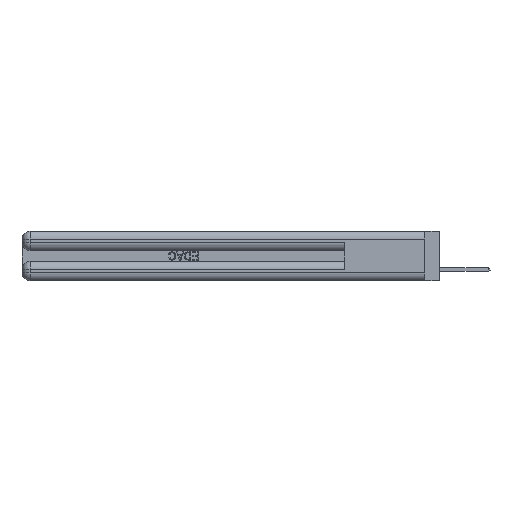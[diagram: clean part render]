
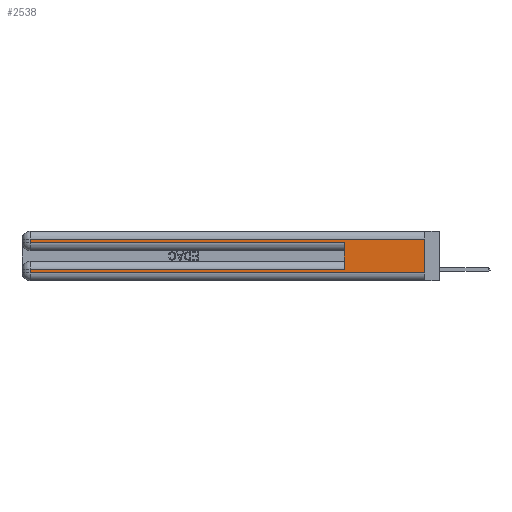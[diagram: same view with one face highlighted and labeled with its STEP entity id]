
A CAD part, left-side view. The second image highlights one B-rep face of the part: STEP entity #2538.
In plain terms, the highlighted planar face has unit normal (-1, 0, 0).
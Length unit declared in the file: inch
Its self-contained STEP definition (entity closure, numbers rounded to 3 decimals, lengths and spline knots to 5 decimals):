
#1200 = CARTESIAN_POINT ( 'NONE',  ( 0., 0., 0.37 ) ) ;
#1521 = CARTESIAN_POINT ( 'NONE',  ( 0., 0.6, 0.285 ) ) ;
#2370 = AXIS2_PLACEMENT_3D ( 'NONE', #34745, #12006, #21709 ) ;
#2538 = ADVANCED_FACE ( 'NONE', ( #9168 ), #5269, .F. ) ;
#3090 = DIRECTION ( 'NONE',  ( 0., 0., -1. ) ) ;
#3160 = DIRECTION ( 'NONE',  ( 0., 1., 0. ) ) ;
#3870 = DIRECTION ( 'NONE',  ( 0., -1., 0. ) ) ;
#5269 = PLANE ( 'NONE',  #2370 ) ;
#5650 = EDGE_CURVE ( 'NONE', #10158, #11535, #15605, .T. ) ;
#6093 = VECTOR ( 'NONE', #3160, 39.37008 ) ;
#6215 = LINE ( 'NONE', #7776, #11859 ) ;
#6504 = LINE ( 'NONE', #20727, #42421 ) ;
#6825 = VERTEX_POINT ( 'NONE', #21568 ) ;
#7388 = DIRECTION ( 'NONE',  ( 0., 1., 0. ) ) ;
#7776 = CARTESIAN_POINT ( 'NONE',  ( 0., 0.6, 0.145 ) ) ;
#9168 = FACE_OUTER_BOUND ( 'NONE', #27084, .T. ) ;
#10158 = VERTEX_POINT ( 'NONE', #32907 ) ;
#10251 = EDGE_CURVE ( 'NONE', #6825, #13430, #14712, .T. ) ;
#10540 = CARTESIAN_POINT ( 'NONE',  ( 0., 2.94, 0.37 ) ) ;
#10787 = CARTESIAN_POINT ( 'NONE',  ( 0., 2.94, 0.31 ) ) ;
#11535 = VERTEX_POINT ( 'NONE', #21443 ) ;
#11615 = DIRECTION ( 'NONE',  ( 0., -1., 0. ) ) ;
#11859 = VECTOR ( 'NONE', #14200, 39.37008 ) ;
#11925 = EDGE_CURVE ( 'NONE', #23346, #28548, #39711, .T. ) ;
#12006 = DIRECTION ( 'NONE',  ( 1., 0., 0. ) ) ;
#12674 = VERTEX_POINT ( 'NONE', #24834 ) ;
#13420 = EDGE_CURVE ( 'NONE', #23346, #11535, #28756, .T. ) ;
#13430 = VERTEX_POINT ( 'NONE', #1521 ) ;
#13829 = EDGE_CURVE ( 'NONE', #41692, #13430, #6215, .T. ) ;
#14200 = DIRECTION ( 'NONE',  ( 0., 0., 1. ) ) ;
#14659 = ORIENTED_EDGE ( 'NONE', *, *, #29208, .T. ) ;
#14712 = LINE ( 'NONE', #39731, #20286 ) ;
#15605 = LINE ( 'NONE', #37679, #32944 ) ;
#15914 = ORIENTED_EDGE ( 'NONE', *, *, #23931, .T. ) ;
#20286 = VECTOR ( 'NONE', #3870, 39.37008 ) ;
#20727 = CARTESIAN_POINT ( 'NONE',  ( 0., 2.94, 0.37 ) ) ;
#21443 = CARTESIAN_POINT ( 'NONE',  ( 0., 0., 0.06 ) ) ;
#21556 = VECTOR ( 'NONE', #3090, 39.37008 ) ;
#21568 = CARTESIAN_POINT ( 'NONE',  ( 0., 2.94, 0.285 ) ) ;
#21709 = DIRECTION ( 'NONE',  ( 0., 0., -1. ) ) ;
#22285 = VECTOR ( 'NONE', #7388, 39.37008 ) ;
#23346 = VERTEX_POINT ( 'NONE', #38727 ) ;
#23931 = EDGE_CURVE ( 'NONE', #28548, #6825, #6504, .T. ) ;
#24834 = CARTESIAN_POINT ( 'NONE',  ( 0., 2.94, 0.085 ) ) ;
#25278 = DIRECTION ( 'NONE',  ( 0., 0., -1. ) ) ;
#25424 = ORIENTED_EDGE ( 'NONE', *, *, #5650, .T. ) ;
#26942 = CARTESIAN_POINT ( 'NONE',  ( 0., 0., 0.31 ) ) ;
#27084 = EDGE_LOOP ( 'NONE', ( #38645, #40670, #15914, #36235, #41682, #14659, #37068, #25424 ) ) ;
#27805 = EDGE_CURVE ( 'NONE', #12674, #10158, #31768, .T. ) ;
#28548 = VERTEX_POINT ( 'NONE', #10787 ) ;
#28756 = LINE ( 'NONE', #1200, #37520 ) ;
#29065 = LINE ( 'NONE', #39039, #6093 ) ;
#29208 = EDGE_CURVE ( 'NONE', #41692, #12674, #29065, .T. ) ;
#31768 = LINE ( 'NONE', #10540, #21556 ) ;
#32907 = CARTESIAN_POINT ( 'NONE',  ( 0., 2.94, 0.06 ) ) ;
#32944 = VECTOR ( 'NONE', #11615, 39.37008 ) ;
#34745 = CARTESIAN_POINT ( 'NONE',  ( 0., 0., 0.37 ) ) ;
#36235 = ORIENTED_EDGE ( 'NONE', *, *, #10251, .T. ) ;
#37068 = ORIENTED_EDGE ( 'NONE', *, *, #27805, .T. ) ;
#37520 = VECTOR ( 'NONE', #40816, 39.37008 ) ;
#37679 = CARTESIAN_POINT ( 'NONE',  ( 0., 0., 0.06 ) ) ;
#38645 = ORIENTED_EDGE ( 'NONE', *, *, #13420, .F. ) ;
#38727 = CARTESIAN_POINT ( 'NONE',  ( 0., 0., 0.31 ) ) ;
#39039 = CARTESIAN_POINT ( 'NONE',  ( 0., 0., 0.085 ) ) ;
#39711 = LINE ( 'NONE', #26942, #22285 ) ;
#39731 = CARTESIAN_POINT ( 'NONE',  ( 0., 0., 0.285 ) ) ;
#40670 = ORIENTED_EDGE ( 'NONE', *, *, #11925, .T. ) ;
#40816 = DIRECTION ( 'NONE',  ( 0., 0., -1. ) ) ;
#41600 = CARTESIAN_POINT ( 'NONE',  ( 0., 0.6, 0.085 ) ) ;
#41682 = ORIENTED_EDGE ( 'NONE', *, *, #13829, .F. ) ;
#41692 = VERTEX_POINT ( 'NONE', #41600 ) ;
#42421 = VECTOR ( 'NONE', #25278, 39.37008 ) ;
